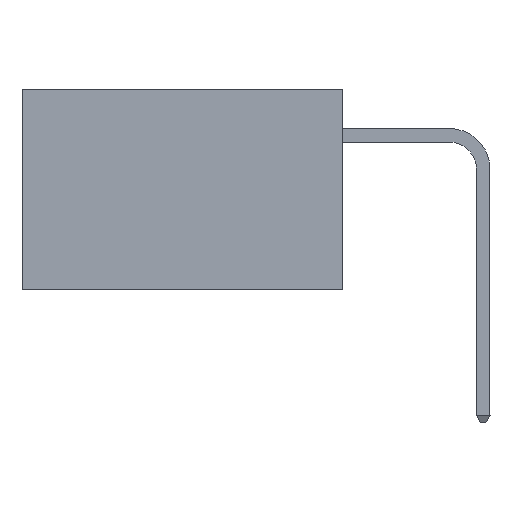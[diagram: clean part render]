
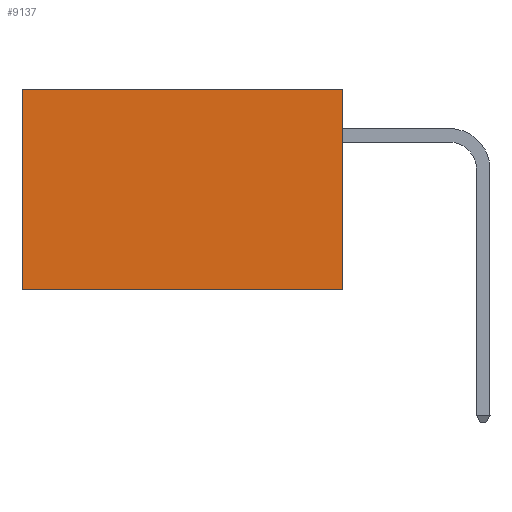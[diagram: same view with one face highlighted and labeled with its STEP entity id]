
A CAD part, left-side view. The second image highlights one B-rep face of the part: STEP entity #9137.
In plain terms, the highlighted planar face has unit normal (-1, 0, 0).
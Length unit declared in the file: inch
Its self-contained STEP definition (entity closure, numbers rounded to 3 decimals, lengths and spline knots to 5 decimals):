
#138 = VECTOR ( 'NONE', #24073, 39.37008 ) ;
#2687 = LINE ( 'NONE', #24105, #7533 ) ;
#4205 = ORIENTED_EDGE ( 'NONE', *, *, #28977, .F. ) ;
#4262 = DIRECTION ( 'NONE',  ( 0., 1., 0. ) ) ;
#4957 = VERTEX_POINT ( 'NONE', #17525 ) ;
#6463 = LINE ( 'NONE', #14750, #138 ) ;
#7170 = EDGE_CURVE ( 'NONE', #8871, #14248, #8698, .T. ) ;
#7359 = CARTESIAN_POINT ( 'NONE',  ( 0.277, 0., -0.37 ) ) ;
#7533 = VECTOR ( 'NONE', #14880, 39.37008 ) ;
#8698 = LINE ( 'NONE', #20629, #26487 ) ;
#8871 = VERTEX_POINT ( 'NONE', #14825 ) ;
#9137 = ADVANCED_FACE ( 'NONE', ( #24528 ), #25163, .F. ) ;
#11290 = CARTESIAN_POINT ( 'NONE',  ( 0.277, 0., -0.37 ) ) ;
#11598 = CARTESIAN_POINT ( 'NONE',  ( 0.277, 0.59, -0.37 ) ) ;
#11934 = LINE ( 'NONE', #7359, #28933 ) ;
#13596 = DIRECTION ( 'NONE',  ( 0., 0., -1. ) ) ;
#14164 = EDGE_CURVE ( 'NONE', #14248, #26314, #6463, .T. ) ;
#14213 = ORIENTED_EDGE ( 'NONE', *, *, #14164, .T. ) ;
#14248 = VERTEX_POINT ( 'NONE', #22067 ) ;
#14355 = EDGE_LOOP ( 'NONE', ( #14213, #4205, #14617, #17865 ) ) ;
#14617 = ORIENTED_EDGE ( 'NONE', *, *, #28892, .F. ) ;
#14750 = CARTESIAN_POINT ( 'NONE',  ( 0.277, 0.59, -0.37 ) ) ;
#14825 = CARTESIAN_POINT ( 'NONE',  ( 0.277, 0., 0. ) ) ;
#14880 = DIRECTION ( 'NONE',  ( 0., 1., 0. ) ) ;
#14919 = AXIS2_PLACEMENT_3D ( 'NONE', #11290, #27489, #13596 ) ;
#17525 = CARTESIAN_POINT ( 'NONE',  ( 0.277, 0., -0.37 ) ) ;
#17865 = ORIENTED_EDGE ( 'NONE', *, *, #7170, .T. ) ;
#20629 = CARTESIAN_POINT ( 'NONE',  ( 0.277, 0., 0. ) ) ;
#22067 = CARTESIAN_POINT ( 'NONE',  ( 0.277, 0.59, 0. ) ) ;
#24073 = DIRECTION ( 'NONE',  ( 0., 0., -1. ) ) ;
#24105 = CARTESIAN_POINT ( 'NONE',  ( 0.277, 0., -0.37 ) ) ;
#24528 = FACE_OUTER_BOUND ( 'NONE', #14355, .T. ) ;
#25163 = PLANE ( 'NONE',  #14919 ) ;
#26158 = DIRECTION ( 'NONE',  ( 0., 0., -1. ) ) ;
#26314 = VERTEX_POINT ( 'NONE', #11598 ) ;
#26487 = VECTOR ( 'NONE', #4262, 39.37008 ) ;
#27489 = DIRECTION ( 'NONE',  ( 1., 0., 0. ) ) ;
#28892 = EDGE_CURVE ( 'NONE', #8871, #4957, #11934, .T. ) ;
#28933 = VECTOR ( 'NONE', #26158, 39.37008 ) ;
#28977 = EDGE_CURVE ( 'NONE', #4957, #26314, #2687, .T. ) ;
